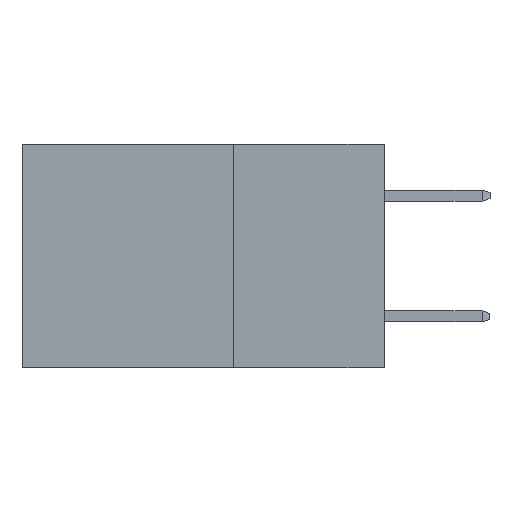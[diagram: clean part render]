
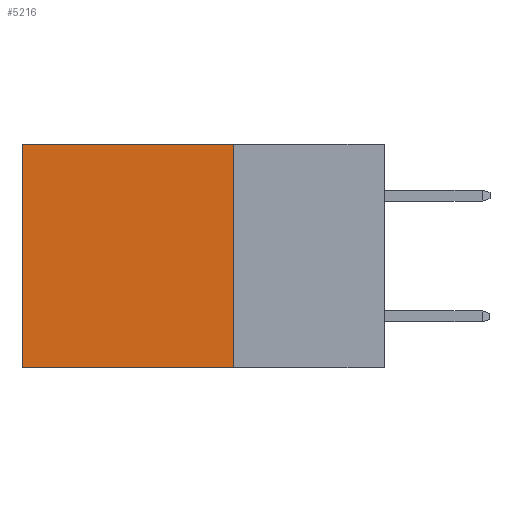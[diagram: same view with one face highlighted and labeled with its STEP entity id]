
A CAD part, left-side view. The second image highlights one B-rep face of the part: STEP entity #5216.
In plain terms, the highlighted planar face has unit normal (-1, 0, 0).
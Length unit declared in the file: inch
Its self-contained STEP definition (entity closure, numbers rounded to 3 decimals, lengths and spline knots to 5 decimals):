
#71 = VECTOR ( 'NONE', #25060, 39.37008 ) ;
#554 = AXIS2_PLACEMENT_3D ( 'NONE', #12998, #9158, #10154 ) ;
#697 = VERTEX_POINT ( 'NONE', #15963 ) ;
#955 = VERTEX_POINT ( 'NONE', #27918 ) ;
#5216 = ADVANCED_FACE ( 'NONE', ( #22255 ), #7448, .F. ) ;
#5221 = VERTEX_POINT ( 'NONE', #14930 ) ;
#5545 = EDGE_CURVE ( 'NONE', #5221, #955, #19794, .T. ) ;
#6033 = LINE ( 'NONE', #22827, #71 ) ;
#6365 = ORIENTED_EDGE ( 'NONE', *, *, #5545, .F. ) ;
#7448 = PLANE ( 'NONE',  #554 ) ;
#8044 = EDGE_CURVE ( 'NONE', #955, #697, #17996, .T. ) ;
#8989 = EDGE_LOOP ( 'NONE', ( #19772, #23455, #6365, #22402 ) ) ;
#9158 = DIRECTION ( 'NONE',  ( 1., 0., 0. ) ) ;
#10154 = DIRECTION ( 'NONE',  ( 0., 0., -1. ) ) ;
#12106 = VECTOR ( 'NONE', #28062, 39.37008 ) ;
#12169 = EDGE_CURVE ( 'NONE', #20991, #697, #6033, .T. ) ;
#12998 = CARTESIAN_POINT ( 'NONE',  ( 0.298, 0.25, 0. ) ) ;
#13199 = VECTOR ( 'NONE', #14448, 39.37008 ) ;
#14448 = DIRECTION ( 'NONE',  ( 0., 1., 0. ) ) ;
#14930 = CARTESIAN_POINT ( 'NONE',  ( 0.298, 0.25, 0. ) ) ;
#15379 = DIRECTION ( 'NONE',  ( 0., 0., -1. ) ) ;
#15963 = CARTESIAN_POINT ( 'NONE',  ( 0.298, 0.6, -0.37 ) ) ;
#17996 = LINE ( 'NONE', #23660, #12106 ) ;
#19730 = LINE ( 'NONE', #25427, #13199 ) ;
#19772 = ORIENTED_EDGE ( 'NONE', *, *, #12169, .T. ) ;
#19794 = LINE ( 'NONE', #28549, #25699 ) ;
#20991 = VERTEX_POINT ( 'NONE', #24787 ) ;
#22255 = FACE_OUTER_BOUND ( 'NONE', #8989, .T. ) ;
#22402 = ORIENTED_EDGE ( 'NONE', *, *, #24715, .T. ) ;
#22827 = CARTESIAN_POINT ( 'NONE',  ( 0.298, 0.6, 0. ) ) ;
#23455 = ORIENTED_EDGE ( 'NONE', *, *, #8044, .F. ) ;
#23660 = CARTESIAN_POINT ( 'NONE',  ( 0.298, 0.25, -0.37 ) ) ;
#24715 = EDGE_CURVE ( 'NONE', #5221, #20991, #19730, .T. ) ;
#24787 = CARTESIAN_POINT ( 'NONE',  ( 0.298, 0.6, 0. ) ) ;
#25060 = DIRECTION ( 'NONE',  ( 0., 0., -1. ) ) ;
#25427 = CARTESIAN_POINT ( 'NONE',  ( 0.298, 0.25, 0. ) ) ;
#25699 = VECTOR ( 'NONE', #15379, 39.37008 ) ;
#27918 = CARTESIAN_POINT ( 'NONE',  ( 0.298, 0.25, -0.37 ) ) ;
#28062 = DIRECTION ( 'NONE',  ( 0., 1., 0. ) ) ;
#28549 = CARTESIAN_POINT ( 'NONE',  ( 0.298, 0.25, 0. ) ) ;
